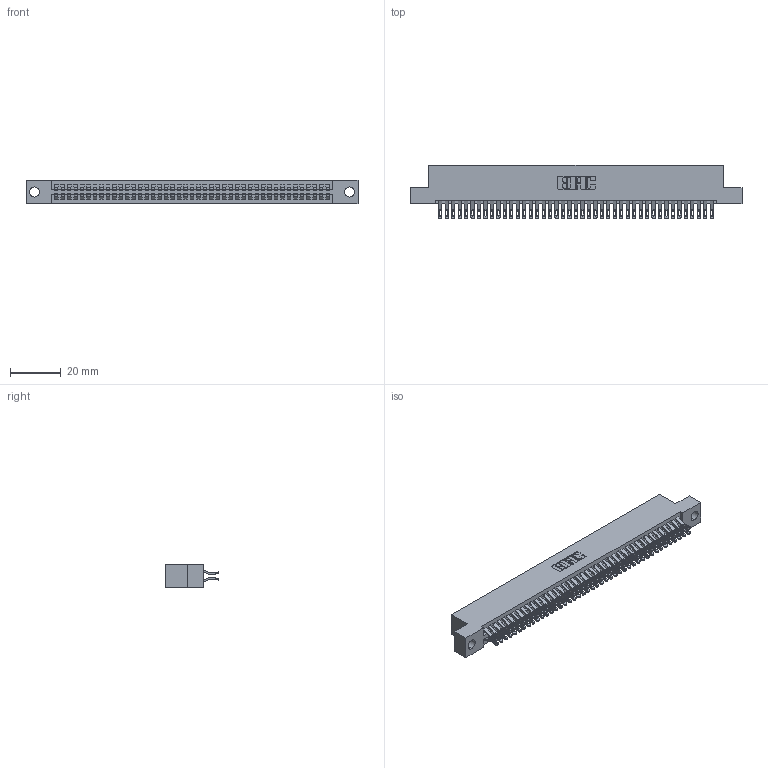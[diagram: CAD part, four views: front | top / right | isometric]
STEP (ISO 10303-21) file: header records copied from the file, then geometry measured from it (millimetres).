
FILE_DESCRIPTION (( 'STEP AP203' ), '1' );
FILE_NAME ('395-086-555-204.STEP', '2018-11-28T21:43:13', ( '' ), ( '' ), 'SwSTEP 2.0', 'SolidWorks 2016', '' );
FILE_SCHEMA (( 'CONFIG_CONTROL_DESIGN' ));
Length unit declared in the file: inch
Products named in the file (3): 345-292-001_555 Tail; 345 Part_Flush Mounting Lugs - 0.156 Dia-TH; 395-086-555-204
Assembly tree (87 placements, depth 2):
  395-086-555-204
    345 Part_Flush Mounting Lugs - 0.156 Dia-TH
    345-292-001_555 Tail  x86
Bounding box: 130.43 x 21.13 x 9.4 mm (x, y, z)
Volume: 12840.9 mm3; surface area: 19683.1 mm2
Topology: 87 solids, 87 shells, 4942 faces, 15563 edges, 10374 vertices
Faces by surface type: plane 2746, cylinder 2196
Entity records: 33933 total; most frequent: CARTESIAN_POINT 5722, ORIENTED_EDGE 5626, DIRECTION 5013, EDGE_CURVE 2813, LINE 2489, VECTOR 2489, VERTEX_POINT 1874, AXIS2_PLACEMENT_3D 1262
